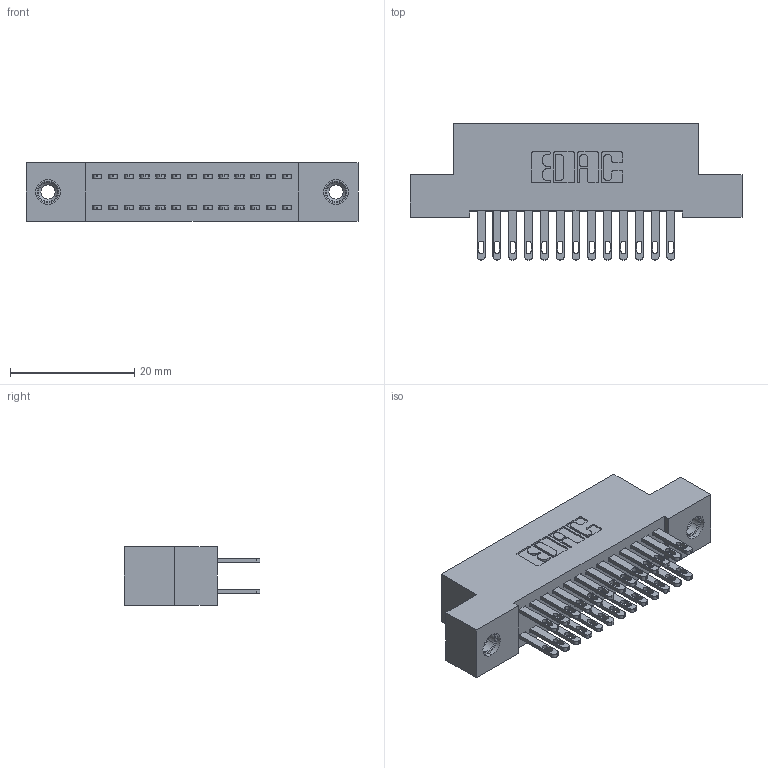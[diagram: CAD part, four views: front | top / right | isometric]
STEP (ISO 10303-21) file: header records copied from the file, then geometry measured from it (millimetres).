
FILE_DESCRIPTION (( 'STEP AP203' ), '1' );
FILE_NAME ('892-026-500-208.STEP', '2020-09-21T14:42:33', ( '' ), ( '' ), 'SwSTEP 2.0', 'SolidWorks 2020', '' );
FILE_SCHEMA (( 'CONFIG_CONTROL_DESIGN' ));
Length unit declared in the file: inch
Products named in the file (4): 345-250-001_345-250-003-102; 345-292-001_345-293-100; 842 Part_TI; 892-026-500-208
Assembly tree (29 placements, depth 2):
  892-026-500-208
    842 Part_TI
    345-292-001_345-293-100  x26
    345-250-001_345-250-003-102  x2
Bounding box: 53.34 x 21.85 x 9.4 mm (x, y, z)
Volume: 4729.1 mm3; surface area: 7242.4 mm2
Topology: 29 solids, 29 shells, 1418 faces, 4257 edges, 2830 vertices
Faces by surface type: plane 878, cylinder 524, cone 12, torus 4
Entity records: 13098 total; most frequent: CARTESIAN_POINT 2185, ORIENTED_EDGE 2114, DIRECTION 1951, EDGE_CURVE 1057, LINE 905, VECTOR 905, VERTEX_POINT 700, AXIS2_PLACEMENT_3D 523
